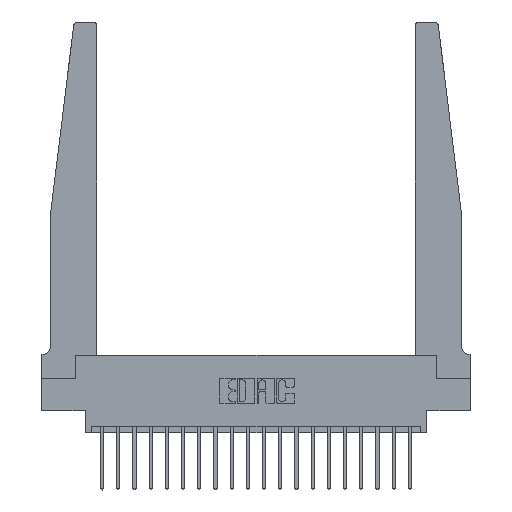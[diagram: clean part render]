
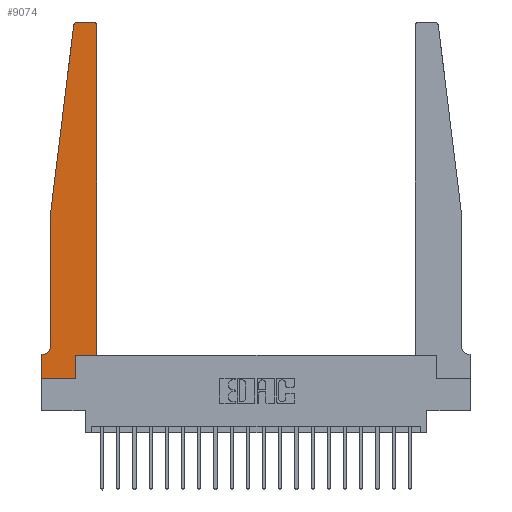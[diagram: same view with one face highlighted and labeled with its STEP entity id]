
A CAD part, top view. The second image highlights one B-rep face of the part: STEP entity #9074.
In plain terms, the highlighted planar face has unit normal (0, 0, 1).
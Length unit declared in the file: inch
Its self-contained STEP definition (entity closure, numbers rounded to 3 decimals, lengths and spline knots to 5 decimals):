
#150 = CARTESIAN_POINT ( 'NONE',  ( 0.065, 1.25, 0.37 ) ) ;
#215 = VERTEX_POINT ( 'NONE', #14849 ) ;
#264 = CIRCLE ( 'NONE', #19476, 0.05 ) ;
#330 = DIRECTION ( 'NONE',  ( 1., 0., 0. ) ) ;
#465 = CARTESIAN_POINT ( 'NONE',  ( 0.395, 2.72, 0.37 ) ) ;
#737 = EDGE_CURVE ( 'NONE', #4945, #15031, #12986, .T. ) ;
#968 = DIRECTION ( 'NONE',  ( -1., 0., 0. ) ) ;
#1057 = AXIS2_PLACEMENT_3D ( 'NONE', #12969, #3305, #14582 ) ;
#1080 = LINE ( 'NONE', #16195, #13445 ) ;
#1233 = CARTESIAN_POINT ( 'NONE',  ( 0., 0.1875, 0.37 ) ) ;
#1299 = VECTOR ( 'NONE', #20904, 39.37008 ) ;
#1463 = VERTEX_POINT ( 'NONE', #12059 ) ;
#1667 = VERTEX_POINT ( 'NONE', #4827 ) ;
#2098 = DIRECTION ( 'NONE',  ( 1., 0., 0. ) ) ;
#2344 = EDGE_CURVE ( 'NONE', #15031, #10448, #20810, .T. ) ;
#2632 = CARTESIAN_POINT ( 'NONE',  ( 0.425, 2.72, 0.37 ) ) ;
#2702 = LINE ( 'NONE', #15123, #6523 ) ;
#2721 = EDGE_CURVE ( 'NONE', #10448, #1667, #6125, .T. ) ;
#2931 = AXIS2_PLACEMENT_3D ( 'NONE', #465, #11736, #2098 ) ;
#3104 = CARTESIAN_POINT ( 'NONE',  ( 0., 0., 0.37 ) ) ;
#3305 = DIRECTION ( 'NONE',  ( 0., 0., 1. ) ) ;
#3341 = CARTESIAN_POINT ( 'NONE',  ( 0.065, 0.1875, 0.37 ) ) ;
#3386 = DIRECTION ( 'NONE',  ( 0., -1., 0. ) ) ;
#3651 = ORIENTED_EDGE ( 'NONE', *, *, #17865, .T. ) ;
#4045 = CARTESIAN_POINT ( 'NONE',  ( 0.395, 2.75, 0.37 ) ) ;
#4239 = VERTEX_POINT ( 'NONE', #17014 ) ;
#4254 = DIRECTION ( 'NONE',  ( 0., 0., 1. ) ) ;
#4717 = VECTOR ( 'NONE', #4994, 39.37008 ) ;
#4827 = CARTESIAN_POINT ( 'NONE',  ( 0.27653, 2.75, 0.37 ) ) ;
#4945 = VERTEX_POINT ( 'NONE', #17131 ) ;
#4994 = DIRECTION ( 'NONE',  ( -1., 0., 0. ) ) ;
#6125 = LINE ( 'NONE', #15966, #1299 ) ;
#6523 = VECTOR ( 'NONE', #16766, 39.37008 ) ;
#6596 = AXIS2_PLACEMENT_3D ( 'NONE', #13890, #4254, #15501 ) ;
#6727 = VERTEX_POINT ( 'NONE', #15088 ) ;
#7181 = ORIENTED_EDGE ( 'NONE', *, *, #2344, .T. ) ;
#7419 = VECTOR ( 'NONE', #11192, 39.37008 ) ;
#7610 = EDGE_CURVE ( 'NONE', #4239, #215, #15469, .T. ) ;
#7750 = DIRECTION ( 'NONE',  ( 0., 1., 0. ) ) ;
#8154 = VERTEX_POINT ( 'NONE', #1233 ) ;
#8208 = VECTOR ( 'NONE', #7750, 39.37008 ) ;
#8276 = ORIENTED_EDGE ( 'NONE', *, *, #7610, .T. ) ;
#8580 = CARTESIAN_POINT ( 'NONE',  ( 0., 0., 0.37 ) ) ;
#9074 = ADVANCED_FACE ( 'NONE', ( #13900 ), #19431, .T. ) ;
#9174 = ORIENTED_EDGE ( 'NONE', *, *, #13438, .T. ) ;
#9373 = EDGE_CURVE ( 'NONE', #1463, #19788, #264, .T. ) ;
#9396 = LINE ( 'NONE', #150, #17478 ) ;
#9497 = LINE ( 'NONE', #3341, #4717 ) ;
#9621 = VECTOR ( 'NONE', #330, 39.37008 ) ;
#10448 = VERTEX_POINT ( 'NONE', #4045 ) ;
#10625 = DIRECTION ( 'NONE',  ( 0., 0., -1. ) ) ;
#10746 = LINE ( 'NONE', #8580, #14010 ) ;
#11036 = ORIENTED_EDGE ( 'NONE', *, *, #19280, .T. ) ;
#11192 = DIRECTION ( 'NONE',  ( -0.122, -0.992, 0. ) ) ;
#11570 = CARTESIAN_POINT ( 'NONE',  ( 0.015, 0.1875, 0.37 ) ) ;
#11736 = DIRECTION ( 'NONE',  ( 0., 0., 1. ) ) ;
#11936 = VERTEX_POINT ( 'NONE', #18244 ) ;
#12059 = CARTESIAN_POINT ( 'NONE',  ( 0.065, 0.2375, 0.37 ) ) ;
#12718 = EDGE_CURVE ( 'NONE', #6727, #11936, #1080, .T. ) ;
#12969 = CARTESIAN_POINT ( 'NONE',  ( 0., 0.1875, 0.37 ) ) ;
#12986 = LINE ( 'NONE', #16372, #8208 ) ;
#13385 = LINE ( 'NONE', #18066, #9621 ) ;
#13438 = EDGE_CURVE ( 'NONE', #215, #1463, #9396, .T. ) ;
#13445 = VECTOR ( 'NONE', #17833, 39.37008 ) ;
#13654 = ORIENTED_EDGE ( 'NONE', *, *, #9373, .T. ) ;
#13890 = CARTESIAN_POINT ( 'NONE',  ( 0.27653, 2.72, 0.37 ) ) ;
#13900 = FACE_OUTER_BOUND ( 'NONE', #16395, .T. ) ;
#14010 = VECTOR ( 'NONE', #18250, 39.37008 ) ;
#14185 = EDGE_CURVE ( 'NONE', #11936, #4945, #13385, .T. ) ;
#14395 = ORIENTED_EDGE ( 'NONE', *, *, #2721, .T. ) ;
#14582 = DIRECTION ( 'NONE',  ( 1., 0., 0. ) ) ;
#14771 = CIRCLE ( 'NONE', #6596, 0.03 ) ;
#14798 = ORIENTED_EDGE ( 'NONE', *, *, #14185, .T. ) ;
#14849 = CARTESIAN_POINT ( 'NONE',  ( 0.065, 1.25, 0.37 ) ) ;
#15031 = VERTEX_POINT ( 'NONE', #2632 ) ;
#15088 = CARTESIAN_POINT ( 'NONE',  ( 0.2605, 0., 0.37 ) ) ;
#15123 = CARTESIAN_POINT ( 'NONE',  ( 0., 0., 0.37 ) ) ;
#15439 = ORIENTED_EDGE ( 'NONE', *, *, #12718, .T. ) ;
#15469 = LINE ( 'NONE', #20921, #7419 ) ;
#15501 = DIRECTION ( 'NONE',  ( 1., 0., 0. ) ) ;
#15966 = CARTESIAN_POINT ( 'NONE',  ( 0.25, 2.75, 0.37 ) ) ;
#16195 = CARTESIAN_POINT ( 'NONE',  ( 0.2605, 0.18, 0.37 ) ) ;
#16372 = CARTESIAN_POINT ( 'NONE',  ( 0.425, 0.18, 0.37 ) ) ;
#16395 = EDGE_LOOP ( 'NONE', ( #14395, #18140, #8276, #9174, #13654, #3651, #11036, #20332, #15439, #14798, #16845, #7181 ) ) ;
#16766 = DIRECTION ( 'NONE',  ( 0., -1., 0. ) ) ;
#16845 = ORIENTED_EDGE ( 'NONE', *, *, #737, .T. ) ;
#17014 = CARTESIAN_POINT ( 'NONE',  ( 0.24675, 2.72367, 0.37 ) ) ;
#17131 = CARTESIAN_POINT ( 'NONE',  ( 0.425, 0.18, 0.37 ) ) ;
#17478 = VECTOR ( 'NONE', #3386, 39.37008 ) ;
#17833 = DIRECTION ( 'NONE',  ( 0., 1., 0. ) ) ;
#17865 = EDGE_CURVE ( 'NONE', #19788, #8154, #9497, .T. ) ;
#18036 = EDGE_CURVE ( 'NONE', #18272, #6727, #10746, .T. ) ;
#18066 = CARTESIAN_POINT ( 'NONE',  ( 0.425, 0.18, 0.37 ) ) ;
#18140 = ORIENTED_EDGE ( 'NONE', *, *, #20071, .T. ) ;
#18244 = CARTESIAN_POINT ( 'NONE',  ( 0.2605, 0.18, 0.37 ) ) ;
#18250 = DIRECTION ( 'NONE',  ( 1., 0., 0. ) ) ;
#18272 = VERTEX_POINT ( 'NONE', #3104 ) ;
#19280 = EDGE_CURVE ( 'NONE', #8154, #18272, #2702, .T. ) ;
#19431 = PLANE ( 'NONE',  #1057 ) ;
#19476 = AXIS2_PLACEMENT_3D ( 'NONE', #20346, #10625, #968 ) ;
#19788 = VERTEX_POINT ( 'NONE', #11570 ) ;
#20071 = EDGE_CURVE ( 'NONE', #1667, #4239, #14771, .T. ) ;
#20332 = ORIENTED_EDGE ( 'NONE', *, *, #18036, .T. ) ;
#20346 = CARTESIAN_POINT ( 'NONE',  ( 0.015, 0.2375, 0.37 ) ) ;
#20810 = CIRCLE ( 'NONE', #2931, 0.03 ) ;
#20904 = DIRECTION ( 'NONE',  ( -1., 0., 0. ) ) ;
#20921 = CARTESIAN_POINT ( 'NONE',  ( 0.065, 1.25, 0.37 ) ) ;
